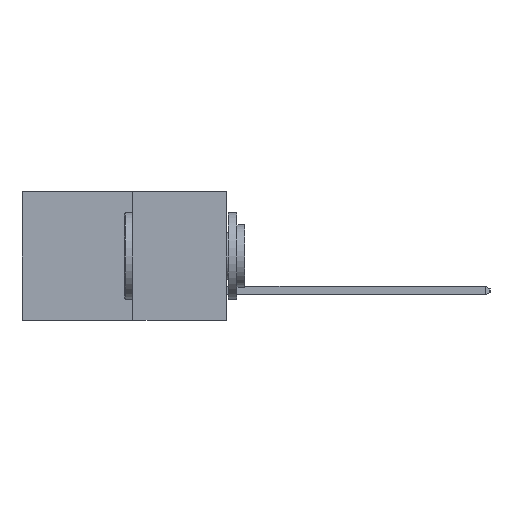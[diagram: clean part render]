
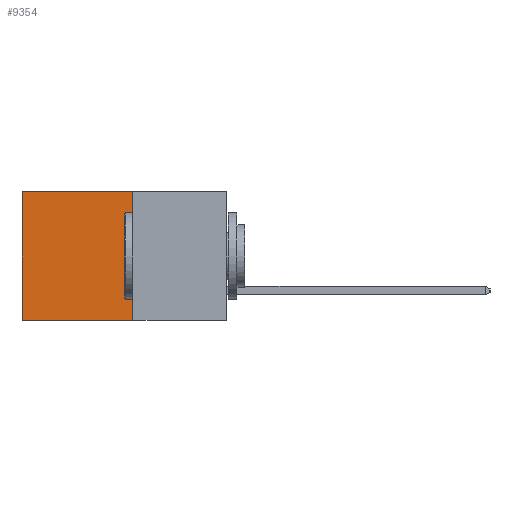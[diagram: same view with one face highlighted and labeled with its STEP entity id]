
A CAD part, left-side view. The second image highlights one B-rep face of the part: STEP entity #9354.
In plain terms, the highlighted planar face has unit normal (-1, 0, 0).
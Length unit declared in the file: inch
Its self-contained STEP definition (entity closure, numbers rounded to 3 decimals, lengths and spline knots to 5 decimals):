
#360 = CARTESIAN_POINT ( 'NONE',  ( 0.277, 0.27, -0.37 ) ) ;
#608 = DIRECTION ( 'NONE',  ( 0., 0., -1. ) ) ;
#686 = DIRECTION ( 'NONE',  ( 1., 0., 0. ) ) ;
#722 = PLANE ( 'NONE',  #13406 ) ;
#1206 = CARTESIAN_POINT ( 'NONE',  ( 0.277, 0.27, -0.37 ) ) ;
#1900 = ORIENTED_EDGE ( 'NONE', *, *, #16010, .T. ) ;
#2319 = LINE ( 'NONE', #17006, #5208 ) ;
#2660 = DIRECTION ( 'NONE',  ( 0., 1., 0. ) ) ;
#3155 = EDGE_CURVE ( 'NONE', #9844, #10426, #8579, .T. ) ;
#3170 = EDGE_LOOP ( 'NONE', ( #1900, #13796, #3693, #10438 ) ) ;
#3196 = LINE ( 'NONE', #11878, #13746 ) ;
#3693 = ORIENTED_EDGE ( 'NONE', *, *, #14525, .F. ) ;
#3755 = CARTESIAN_POINT ( 'NONE',  ( 0.277, 0.27, 0. ) ) ;
#4373 = LINE ( 'NONE', #15334, #8137 ) ;
#5208 = VECTOR ( 'NONE', #10356, 39.37008 ) ;
#5824 = DIRECTION ( 'NONE',  ( 0., 0., -1. ) ) ;
#7460 = VERTEX_POINT ( 'NONE', #10558 ) ;
#8137 = VECTOR ( 'NONE', #5824, 39.37008 ) ;
#8579 = LINE ( 'NONE', #3755, #11737 ) ;
#9354 = ADVANCED_FACE ( 'NONE', ( #12199 ), #722, .F. ) ;
#9844 = VERTEX_POINT ( 'NONE', #16350 ) ;
#10356 = DIRECTION ( 'NONE',  ( 0., 0., -1. ) ) ;
#10426 = VERTEX_POINT ( 'NONE', #17580 ) ;
#10438 = ORIENTED_EDGE ( 'NONE', *, *, #3155, .T. ) ;
#10558 = CARTESIAN_POINT ( 'NONE',  ( 0.277, 0.59, -0.37 ) ) ;
#10783 = EDGE_CURVE ( 'NONE', #17295, #7460, #3196, .T. ) ;
#11737 = VECTOR ( 'NONE', #2660, 39.37008 ) ;
#11878 = CARTESIAN_POINT ( 'NONE',  ( 0.277, 0.27, -0.37 ) ) ;
#12199 = FACE_OUTER_BOUND ( 'NONE', #3170, .T. ) ;
#13228 = DIRECTION ( 'NONE',  ( 0., 1., 0. ) ) ;
#13406 = AXIS2_PLACEMENT_3D ( 'NONE', #1206, #686, #608 ) ;
#13746 = VECTOR ( 'NONE', #13228, 39.37008 ) ;
#13796 = ORIENTED_EDGE ( 'NONE', *, *, #10783, .F. ) ;
#14525 = EDGE_CURVE ( 'NONE', #9844, #17295, #4373, .T. ) ;
#15334 = CARTESIAN_POINT ( 'NONE',  ( 0.277, 0.27, -0.37 ) ) ;
#16010 = EDGE_CURVE ( 'NONE', #10426, #7460, #2319, .T. ) ;
#16350 = CARTESIAN_POINT ( 'NONE',  ( 0.277, 0.27, 0. ) ) ;
#17006 = CARTESIAN_POINT ( 'NONE',  ( 0.277, 0.59, -0.37 ) ) ;
#17295 = VERTEX_POINT ( 'NONE', #360 ) ;
#17580 = CARTESIAN_POINT ( 'NONE',  ( 0.277, 0.59, 0. ) ) ;
